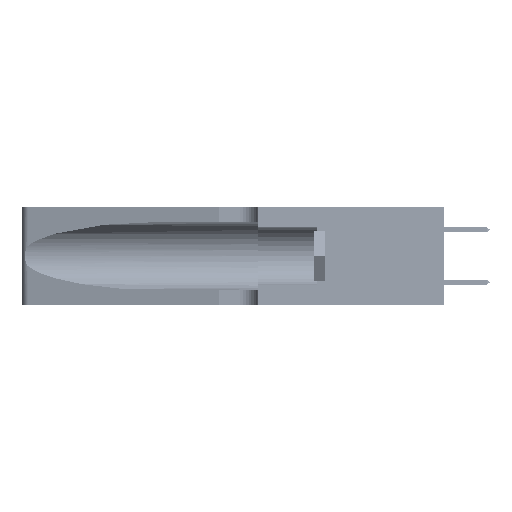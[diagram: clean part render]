
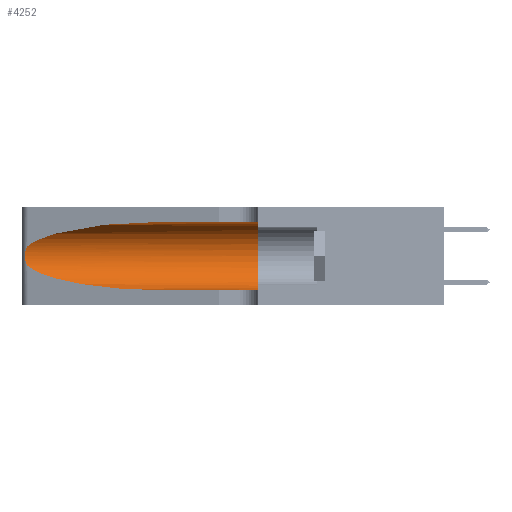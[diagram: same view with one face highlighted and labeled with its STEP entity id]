
A CAD part, left-side view. The second image highlights one B-rep face of the part: STEP entity #4252.
In plain terms, the highlighted cylindrical face has radius 3.308 mm (diameter 6.617 mm), a partial arc.
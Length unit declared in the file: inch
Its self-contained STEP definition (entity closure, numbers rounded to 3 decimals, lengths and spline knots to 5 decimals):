
#26 = EDGE_CURVE ( 'NONE', #39123, #16269, #20891, .T. ) ;
#444 = CARTESIAN_POINT ( 'NONE',  ( 0.2373, 1.15595, 0.28018 ) ) ;
#652 = EDGE_CURVE ( 'NONE', #20664, #8839, #43926, .T. ) ;
#2795 = CARTESIAN_POINT ( 'NONE',  ( 0.25856, 1.23593, 0.16098 ) ) ;
#4252 = ADVANCED_FACE ( 'NONE', ( #32649 ), #33148, .F. ) ;
#4905 = CARTESIAN_POINT ( 'NONE',  ( 0.18966, 0.96281, 0.05475 ) ) ;
#6803 = EDGE_CURVE ( 'NONE', #16269, #8486, #22309, .T. ) ;
#7211 = CARTESIAN_POINT ( 'NONE',  ( 0.1305, 0.72297, 0.31525 ) ) ;
#7241 = EDGE_CURVE ( 'NONE', #39123, #20664, #37586, .T. ) ;
#8486 = VERTEX_POINT ( 'NONE', #29036 ) ;
#8839 = VERTEX_POINT ( 'NONE', #45640 ) ;
#9883 = VERTEX_POINT ( 'NONE', #26147 ) ;
#11920 = LINE ( 'NONE', #18232, #39387 ) ;
#11964 = CARTESIAN_POINT ( 'NONE',  ( 0.25487, 1.22718, 0.14631 ) ) ;
#12141 = EDGE_CURVE ( 'NONE', #8486, #9883, #44436, .T. ) ;
#13021 = CARTESIAN_POINT ( 'NONE',  ( 0.26075, 1.23896, 0.19203 ) ) ;
#16205 = CARTESIAN_POINT ( 'NONE',  ( 0.1305, 1.61858, 0.185 ) ) ;
#16269 = VERTEX_POINT ( 'NONE', #35402 ) ;
#17258 = CARTESIAN_POINT ( 'NONE',  ( 0.25639, 1.23184, 0.21858 ) ) ;
#18232 = CARTESIAN_POINT ( 'NONE',  ( 0.1305, 1.61858, 0.05475 ) ) ;
#18504 = AXIS2_PLACEMENT_3D ( 'NONE', #42737, #21300, #36168 ) ;
#18508 = CARTESIAN_POINT ( 'NONE',  ( 0.25487, 1.22718, 0.22369 ) ) ;
#18532 = DIRECTION ( 'NONE',  ( 0., -1., 0. ) ) ;
#19189 = CARTESIAN_POINT ( 'NONE',  ( 0.2373, 1.15595, 0.08982 ) ) ;
#19460 = AXIS2_PLACEMENT_3D ( 'NONE', #16205, #31721, #36573 ) ;
#20419 = EDGE_LOOP ( 'NONE', ( #20619, #35883, #27779, #41883, #41345, #42972 ) ) ;
#20619 = ORIENTED_EDGE ( 'NONE', *, *, #26, .T. ) ;
#20664 = VERTEX_POINT ( 'NONE', #40892 ) ;
#20891 =( BOUNDED_CURVE ( )  B_SPLINE_CURVE ( 3, ( #7211, #43072, #444, #18508 ),
 .UNSPECIFIED., .F., .F. ) 
 B_SPLINE_CURVE_WITH_KNOTS ( ( 4, 4 ),
 ( 1.5708, 2.84003 ),
 .UNSPECIFIED. ) 
 CURVE ( )  GEOMETRIC_REPRESENTATION_ITEM ( )  RATIONAL_B_SPLINE_CURVE ( ( 1., 0.87, 0.87, 1. ) ) 
 REPRESENTATION_ITEM ( '' )  );
#21300 = DIRECTION ( 'NONE',  ( 0., 1., 0. ) ) ;
#22309 = B_SPLINE_CURVE_WITH_KNOTS ( 'NONE', 3,
 ( #41971, #45574, #17258, #45727, #27402, #24272, #13021, #24119, #41675, #2795, #30869, #45263, #27867, #23816 ),
 .UNSPECIFIED., .F., .F.,
 ( 4, 2, 2, 2, 2, 2, 4 ),
 ( 0., 0.00027, 0.00053, 0.00107, 0.0016, 0.00187, 0.00214 ),
 .UNSPECIFIED. ) ;
#23453 = DIRECTION ( 'NONE',  ( 0., -1., 0. ) ) ;
#23816 = CARTESIAN_POINT ( 'NONE',  ( 0.25487, 1.22718, 0.14631 ) ) ;
#24119 = CARTESIAN_POINT ( 'NONE',  ( 0.26075, 1.23896, 0.178 ) ) ;
#24272 = CARTESIAN_POINT ( 'NONE',  ( 0.26018, 1.23835, 0.19895 ) ) ;
#24675 = VECTOR ( 'NONE', #23453, 39.37008 ) ;
#26034 = CARTESIAN_POINT ( 'NONE',  ( 0.1305, 0.72297, 0.31525 ) ) ;
#26147 = CARTESIAN_POINT ( 'NONE',  ( 0.1305, 0.72297, 0.05475 ) ) ;
#26368 = CARTESIAN_POINT ( 'NONE',  ( 0.1305, 0.72297, 0.05475 ) ) ;
#27402 = CARTESIAN_POINT ( 'NONE',  ( 0.25854, 1.2359, 0.20912 ) ) ;
#27779 = ORIENTED_EDGE ( 'NONE', *, *, #12141, .T. ) ;
#27867 = CARTESIAN_POINT ( 'NONE',  ( 0.25555, 1.22993, 0.14849 ) ) ;
#29036 = CARTESIAN_POINT ( 'NONE',  ( 0.25487, 1.22718, 0.14631 ) ) ;
#30869 = CARTESIAN_POINT ( 'NONE',  ( 0.25789, 1.23486, 0.15765 ) ) ;
#30964 = CARTESIAN_POINT ( 'NONE',  ( 0.1305, 1.61858, 0.31525 ) ) ;
#31721 = DIRECTION ( 'NONE',  ( 0., -1., 0. ) ) ;
#32649 = FACE_OUTER_BOUND ( 'NONE', #20419, .T. ) ;
#33148 = CYLINDRICAL_SURFACE ( 'NONE', #19460, 0.13025 ) ;
#35402 = CARTESIAN_POINT ( 'NONE',  ( 0.25487, 1.22718, 0.22369 ) ) ;
#35883 = ORIENTED_EDGE ( 'NONE', *, *, #6803, .T. ) ;
#36168 = DIRECTION ( 'NONE',  ( 0., 0., 1. ) ) ;
#36573 = DIRECTION ( 'NONE',  ( 0., 0., -1. ) ) ;
#37586 = LINE ( 'NONE', #30964, #24675 ) ;
#39123 = VERTEX_POINT ( 'NONE', #26034 ) ;
#39387 = VECTOR ( 'NONE', #18532, 39.37008 ) ;
#40892 = CARTESIAN_POINT ( 'NONE',  ( 0.1305, 0.35, 0.31525 ) ) ;
#41235 = EDGE_CURVE ( 'NONE', #9883, #8839, #11920, .T. ) ;
#41345 = ORIENTED_EDGE ( 'NONE', *, *, #652, .F. ) ;
#41675 = CARTESIAN_POINT ( 'NONE',  ( 0.26017, 1.23833, 0.17102 ) ) ;
#41883 = ORIENTED_EDGE ( 'NONE', *, *, #41235, .T. ) ;
#41971 = CARTESIAN_POINT ( 'NONE',  ( 0.25487, 1.22718, 0.22369 ) ) ;
#42737 = CARTESIAN_POINT ( 'NONE',  ( 0.1305, 0.35, 0.185 ) ) ;
#42972 = ORIENTED_EDGE ( 'NONE', *, *, #7241, .F. ) ;
#43072 = CARTESIAN_POINT ( 'NONE',  ( 0.18966, 0.96281, 0.31525 ) ) ;
#43926 = CIRCLE ( 'NONE', #18504, 0.13025 ) ;
#44436 =( BOUNDED_CURVE ( )  B_SPLINE_CURVE ( 3, ( #11964, #19189, #4905, #26368 ),
 .UNSPECIFIED., .F., .T. ) 
 B_SPLINE_CURVE_WITH_KNOTS ( ( 4, 4 ),
 ( 3.44316, 4.71239 ),
 .UNSPECIFIED. ) 
 CURVE ( )  GEOMETRIC_REPRESENTATION_ITEM ( )  RATIONAL_B_SPLINE_CURVE ( ( 1., 0.87, 0.87, 1. ) ) 
 REPRESENTATION_ITEM ( '' )  );
#45263 = CARTESIAN_POINT ( 'NONE',  ( 0.25639, 1.23186, 0.15144 ) ) ;
#45574 = CARTESIAN_POINT ( 'NONE',  ( 0.25555, 1.22994, 0.2215 ) ) ;
#45640 = CARTESIAN_POINT ( 'NONE',  ( 0.1305, 0.35, 0.05475 ) ) ;
#45727 = CARTESIAN_POINT ( 'NONE',  ( 0.25787, 1.23484, 0.2124 ) ) ;
